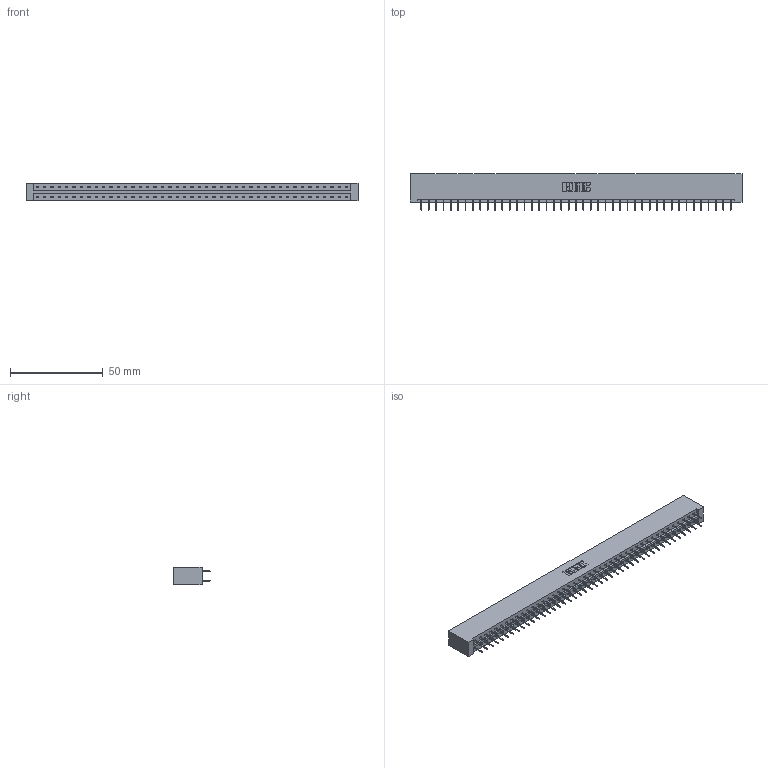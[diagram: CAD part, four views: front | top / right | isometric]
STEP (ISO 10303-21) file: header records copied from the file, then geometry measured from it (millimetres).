
FILE_DESCRIPTION (( 'STEP AP203' ), '1' );
FILE_NAME ('833-086-524-201.STEP', '2020-06-06T03:08:08', ( '' ), ( '' ), 'SwSTEP 2.0', 'SolidWorks 2020', '' );
FILE_SCHEMA (( 'CONFIG_CONTROL_DESIGN' ));
Length unit declared in the file: inch
Products named in the file (3): 833 Part_Lugless; 345-292-001_345-293-124; 833-086-524-201
Assembly tree (87 placements, depth 2):
  833-086-524-201
    833 Part_Lugless
    345-292-001_345-293-124  x86
Bounding box: 178.64 x 19.69 x 9.4 mm (x, y, z)
Volume: 18749.4 mm3; surface area: 21810.9 mm2
Topology: 87 solids, 87 shells, 4922 faces, 13961 edges, 8962 vertices
Faces by surface type: plane 3678, cylinder 1244
Entity records: 27331 total; most frequent: CARTESIAN_POINT 4526, ORIENTED_EDGE 4462, DIRECTION 3859, EDGE_CURVE 2231, LINE 2115, VECTOR 2115, VERTEX_POINT 1482, AXIS2_PLACEMENT_3D 872
